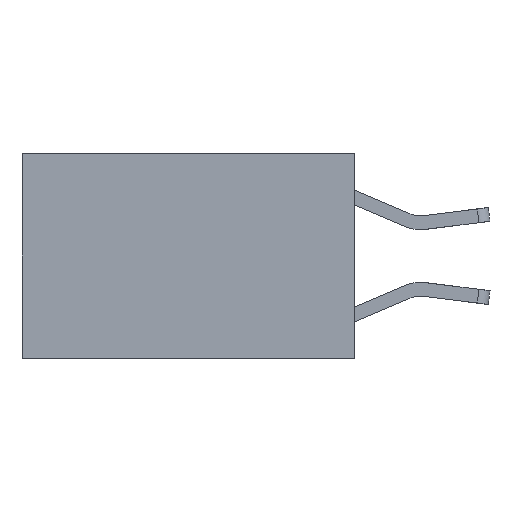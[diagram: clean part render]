
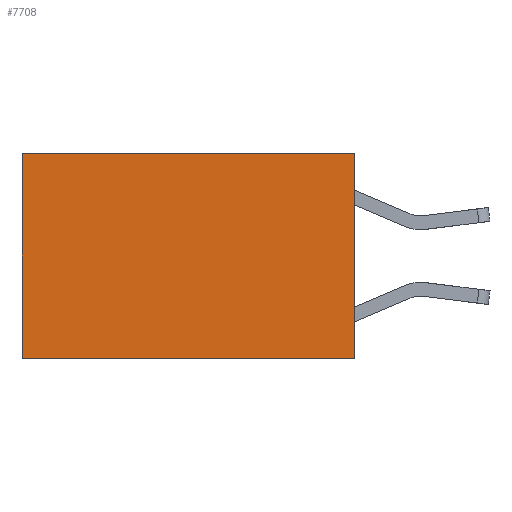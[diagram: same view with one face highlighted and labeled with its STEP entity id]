
A CAD part, left-side view. The second image highlights one B-rep face of the part: STEP entity #7708.
In plain terms, the highlighted planar face has unit normal (-1, 0, 0).
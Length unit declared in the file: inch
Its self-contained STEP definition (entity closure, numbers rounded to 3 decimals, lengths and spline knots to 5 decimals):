
#214 = ORIENTED_EDGE ( 'NONE', *, *, #7662, .F. ) ;
#505 = VERTEX_POINT ( 'NONE', #7526 ) ;
#760 = AXIS2_PLACEMENT_3D ( 'NONE', #968, #922, #2188 ) ;
#849 = LINE ( 'NONE', #7404, #1217 ) ;
#922 = DIRECTION ( 'NONE',  ( 1., 0., 0. ) ) ;
#968 = CARTESIAN_POINT ( 'NONE',  ( 0.2625, 0., 0. ) ) ;
#1025 = VERTEX_POINT ( 'NONE', #7302 ) ;
#1098 = ORIENTED_EDGE ( 'NONE', *, *, #3305, .T. ) ;
#1217 = VECTOR ( 'NONE', #1605, 39.37008 ) ;
#1605 = DIRECTION ( 'NONE',  ( 0., 0., -1. ) ) ;
#1652 = EDGE_CURVE ( 'NONE', #4028, #1025, #849, .T. ) ;
#2052 = EDGE_LOOP ( 'NONE', ( #2161, #214, #4096, #1098 ) ) ;
#2161 = ORIENTED_EDGE ( 'NONE', *, *, #6558, .T. ) ;
#2164 = CARTESIAN_POINT ( 'NONE',  ( 0.2625, 0., 0. ) ) ;
#2188 = DIRECTION ( 'NONE',  ( 0., 0., -1. ) ) ;
#2265 = LINE ( 'NONE', #6796, #6028 ) ;
#3305 = EDGE_CURVE ( 'NONE', #4028, #505, #3803, .T. ) ;
#3379 = PLANE ( 'NONE',  #760 ) ;
#3803 = LINE ( 'NONE', #2164, #4197 ) ;
#4028 = VERTEX_POINT ( 'NONE', #6417 ) ;
#4096 = ORIENTED_EDGE ( 'NONE', *, *, #1652, .F. ) ;
#4138 = LINE ( 'NONE', #6720, #8061 ) ;
#4197 = VECTOR ( 'NONE', #6085, 39.37008 ) ;
#5425 = DIRECTION ( 'NONE',  ( 0., 1., 0. ) ) ;
#5582 = DIRECTION ( 'NONE',  ( 0., 0., -1. ) ) ;
#6028 = VECTOR ( 'NONE', #5582, 39.37008 ) ;
#6085 = DIRECTION ( 'NONE',  ( 0., 1., 0. ) ) ;
#6417 = CARTESIAN_POINT ( 'NONE',  ( 0.2625, 0., 0. ) ) ;
#6558 = EDGE_CURVE ( 'NONE', #505, #7376, #2265, .T. ) ;
#6685 = FACE_OUTER_BOUND ( 'NONE', #2052, .T. ) ;
#6720 = CARTESIAN_POINT ( 'NONE',  ( 0.2625, 0., -0.37 ) ) ;
#6796 = CARTESIAN_POINT ( 'NONE',  ( 0.2625, 0.6, 0. ) ) ;
#7302 = CARTESIAN_POINT ( 'NONE',  ( 0.2625, 0., -0.37 ) ) ;
#7376 = VERTEX_POINT ( 'NONE', #8133 ) ;
#7404 = CARTESIAN_POINT ( 'NONE',  ( 0.2625, 0., 0. ) ) ;
#7526 = CARTESIAN_POINT ( 'NONE',  ( 0.2625, 0.6, 0. ) ) ;
#7662 = EDGE_CURVE ( 'NONE', #1025, #7376, #4138, .T. ) ;
#7708 = ADVANCED_FACE ( 'NONE', ( #6685 ), #3379, .F. ) ;
#8061 = VECTOR ( 'NONE', #5425, 39.37008 ) ;
#8133 = CARTESIAN_POINT ( 'NONE',  ( 0.2625, 0.6, -0.37 ) ) ;
